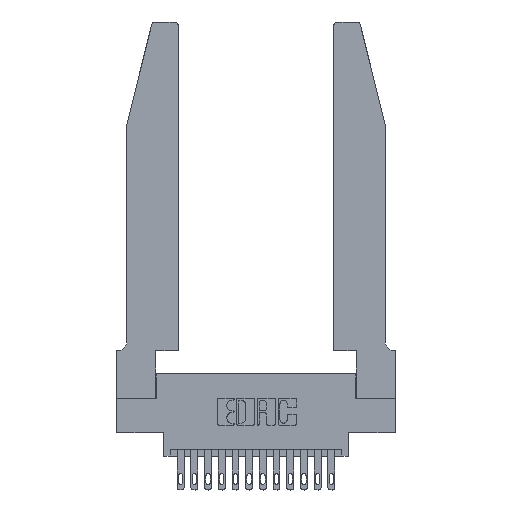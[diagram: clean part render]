
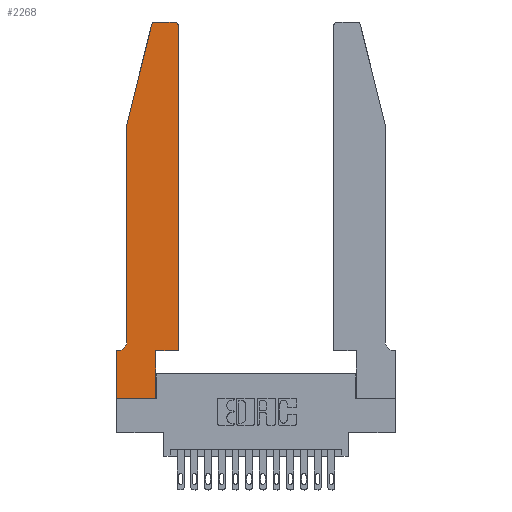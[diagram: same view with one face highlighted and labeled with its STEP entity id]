
A CAD part, top view. The second image highlights one B-rep face of the part: STEP entity #2268.
In plain terms, the highlighted planar face has unit normal (0, 0, 1).
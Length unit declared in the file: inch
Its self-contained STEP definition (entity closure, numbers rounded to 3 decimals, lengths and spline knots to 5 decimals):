
#92 = DIRECTION ( 'NONE',  ( 0., 0., 1. ) ) ;
#184 = ORIENTED_EDGE ( 'NONE', *, *, #8042, .T. ) ;
#872 = ORIENTED_EDGE ( 'NONE', *, *, #10988, .T. ) ;
#1040 = VECTOR ( 'NONE', #16801, 39.37008 ) ;
#1099 = DIRECTION ( 'NONE',  ( 1., 0., 0. ) ) ;
#1201 = EDGE_CURVE ( 'NONE', #16765, #8810, #13561, .T. ) ;
#1229 = DIRECTION ( 'NONE',  ( -1., 0., 0. ) ) ;
#1458 = DIRECTION ( 'NONE',  ( 1., 0., 0. ) ) ;
#1979 = AXIS2_PLACEMENT_3D ( 'NONE', #12449, #15235, #1229 ) ;
#2033 = EDGE_LOOP ( 'NONE', ( #11758, #17235, #184, #8457, #3432, #6998, #6655, #3687, #8711, #6825, #872, #7220 ) ) ;
#2268 = ADVANCED_FACE ( 'NONE', ( #6787 ), #9186, .T. ) ;
#2339 = EDGE_CURVE ( 'NONE', #12014, #3816, #12275, .T. ) ;
#2723 = CARTESIAN_POINT ( 'NONE',  ( 0.4205, 2.75, 0.37 ) ) ;
#2742 = CARTESIAN_POINT ( 'NONE',  ( 0.4505, 0.35, 0.37 ) ) ;
#2926 = EDGE_CURVE ( 'NONE', #8810, #10530, #14921, .T. ) ;
#3192 = AXIS2_PLACEMENT_3D ( 'NONE', #13345, #7558, #4908 ) ;
#3237 = AXIS2_PLACEMENT_3D ( 'NONE', #14167, #92, #1458 ) ;
#3383 = VECTOR ( 'NONE', #9747, 39.37008 ) ;
#3432 = ORIENTED_EDGE ( 'NONE', *, *, #2339, .T. ) ;
#3562 = CARTESIAN_POINT ( 'NONE',  ( 0.0755, 0.35, 0.37 ) ) ;
#3647 = CARTESIAN_POINT ( 'NONE',  ( 0., 0.35, 0.37 ) ) ;
#3648 = LINE ( 'NONE', #8197, #14235 ) ;
#3687 = ORIENTED_EDGE ( 'NONE', *, *, #1201, .T. ) ;
#3816 = VERTEX_POINT ( 'NONE', #4847 ) ;
#4797 = EDGE_CURVE ( 'NONE', #3816, #5520, #5380, .T. ) ;
#4847 = CARTESIAN_POINT ( 'NONE',  ( 0.0055, 0.35, 0.37 ) ) ;
#4908 = DIRECTION ( 'NONE',  ( 1., 0., 0. ) ) ;
#5380 = LINE ( 'NONE', #3562, #17283 ) ;
#5520 = VERTEX_POINT ( 'NONE', #7675 ) ;
#6226 = LINE ( 'NONE', #16584, #9998 ) ;
#6383 = DIRECTION ( 'NONE',  ( -1., 0., 0. ) ) ;
#6390 = EDGE_CURVE ( 'NONE', #12432, #17370, #14367, .T. ) ;
#6594 = DIRECTION ( 'NONE',  ( 0., 0., 1. ) ) ;
#6602 = VERTEX_POINT ( 'NONE', #9844 ) ;
#6655 = ORIENTED_EDGE ( 'NONE', *, *, #17991, .T. ) ;
#6787 = FACE_OUTER_BOUND ( 'NONE', #2033, .T. ) ;
#6825 = ORIENTED_EDGE ( 'NONE', *, *, #15756, .T. ) ;
#6895 = CARTESIAN_POINT ( 'NONE',  ( 0.2865, 0.35, 0.37 ) ) ;
#6998 = ORIENTED_EDGE ( 'NONE', *, *, #4797, .T. ) ;
#7220 = ORIENTED_EDGE ( 'NONE', *, *, #6390, .T. ) ;
#7558 = DIRECTION ( 'NONE',  ( 0., 0., 1. ) ) ;
#7675 = CARTESIAN_POINT ( 'NONE',  ( 0., 0.35, 0.37 ) ) ;
#8042 = EDGE_CURVE ( 'NONE', #8714, #6602, #9462, .T. ) ;
#8156 = DIRECTION ( 'NONE',  ( 1., 0., 0. ) ) ;
#8197 = CARTESIAN_POINT ( 'NONE',  ( 0.0755, 2., 0.37 ) ) ;
#8437 = DIRECTION ( 'NONE',  ( 0., -1., 0. ) ) ;
#8457 = ORIENTED_EDGE ( 'NONE', *, *, #12025, .T. ) ;
#8711 = ORIENTED_EDGE ( 'NONE', *, *, #2926, .T. ) ;
#8714 = VERTEX_POINT ( 'NONE', #14118 ) ;
#8810 = VERTEX_POINT ( 'NONE', #10510 ) ;
#9011 = CIRCLE ( 'NONE', #3237, 0.03 ) ;
#9186 = PLANE ( 'NONE',  #16751 ) ;
#9462 = LINE ( 'NONE', #15212, #17379 ) ;
#9611 = DIRECTION ( 'NONE',  ( 0., -1., 0. ) ) ;
#9747 = DIRECTION ( 'NONE',  ( 1., 0., 0. ) ) ;
#9813 = VECTOR ( 'NONE', #1099, 39.37008 ) ;
#9817 = EDGE_CURVE ( 'NONE', #14340, #8714, #9011, .T. ) ;
#9844 = CARTESIAN_POINT ( 'NONE',  ( 0.0755, 2., 0.37 ) ) ;
#9998 = VECTOR ( 'NONE', #12687, 39.37008 ) ;
#10510 = CARTESIAN_POINT ( 'NONE',  ( 0.2865, 0., 0.37 ) ) ;
#10530 = VERTEX_POINT ( 'NONE', #12834 ) ;
#10717 = DIRECTION ( 'NONE',  ( -0.239, -0.971, 0. ) ) ;
#10988 = EDGE_CURVE ( 'NONE', #16265, #12432, #12936, .T. ) ;
#11128 = CARTESIAN_POINT ( 'NONE',  ( 0., 0., 0.37 ) ) ;
#11173 = VECTOR ( 'NONE', #18281, 39.37008 ) ;
#11206 = CARTESIAN_POINT ( 'NONE',  ( 0., 0., 0.37 ) ) ;
#11302 = VECTOR ( 'NONE', #8437, 39.37008 ) ;
#11758 = ORIENTED_EDGE ( 'NONE', *, *, #14048, .T. ) ;
#12013 = CARTESIAN_POINT ( 'NONE',  ( 0.284, 2.75, 0.37 ) ) ;
#12014 = VERTEX_POINT ( 'NONE', #17066 ) ;
#12025 = EDGE_CURVE ( 'NONE', #6602, #12014, #3648, .T. ) ;
#12275 = CIRCLE ( 'NONE', #1979, 0.07 ) ;
#12432 = VERTEX_POINT ( 'NONE', #17805 ) ;
#12449 = CARTESIAN_POINT ( 'NONE',  ( 0.0055, 0.42, 0.37 ) ) ;
#12687 = DIRECTION ( 'NONE',  ( -1., 0., 0. ) ) ;
#12834 = CARTESIAN_POINT ( 'NONE',  ( 0.2865, 0.35, 0.37 ) ) ;
#12936 = LINE ( 'NONE', #2742, #1040 ) ;
#13345 = CARTESIAN_POINT ( 'NONE',  ( 0.4205, 2.72, 0.37 ) ) ;
#13561 = LINE ( 'NONE', #15042, #9813 ) ;
#13671 = CARTESIAN_POINT ( 'NONE',  ( 0.4505, 0.35, 0.37 ) ) ;
#14048 = EDGE_CURVE ( 'NONE', #17370, #14340, #6226, .T. ) ;
#14118 = CARTESIAN_POINT ( 'NONE',  ( 0.25487, 2.72718, 0.37 ) ) ;
#14167 = CARTESIAN_POINT ( 'NONE',  ( 0.284, 2.72, 0.37 ) ) ;
#14235 = VECTOR ( 'NONE', #9611, 39.37008 ) ;
#14340 = VERTEX_POINT ( 'NONE', #12013 ) ;
#14367 = CIRCLE ( 'NONE', #3192, 0.03 ) ;
#14396 = LINE ( 'NONE', #18189, #3383 ) ;
#14921 = LINE ( 'NONE', #6895, #11173 ) ;
#15042 = CARTESIAN_POINT ( 'NONE',  ( 0., 0., 0.37 ) ) ;
#15212 = CARTESIAN_POINT ( 'NONE',  ( 0.0755, 2., 0.37 ) ) ;
#15235 = DIRECTION ( 'NONE',  ( 0., 0., -1. ) ) ;
#15520 = LINE ( 'NONE', #11206, #11302 ) ;
#15756 = EDGE_CURVE ( 'NONE', #10530, #16265, #14396, .T. ) ;
#16265 = VERTEX_POINT ( 'NONE', #13671 ) ;
#16584 = CARTESIAN_POINT ( 'NONE',  ( 0.2605, 2.75, 0.37 ) ) ;
#16751 = AXIS2_PLACEMENT_3D ( 'NONE', #3647, #6594, #8156 ) ;
#16765 = VERTEX_POINT ( 'NONE', #11128 ) ;
#16801 = DIRECTION ( 'NONE',  ( 0., 1., 0. ) ) ;
#17066 = CARTESIAN_POINT ( 'NONE',  ( 0.0755, 0.42, 0.37 ) ) ;
#17235 = ORIENTED_EDGE ( 'NONE', *, *, #9817, .T. ) ;
#17283 = VECTOR ( 'NONE', #6383, 39.37008 ) ;
#17370 = VERTEX_POINT ( 'NONE', #2723 ) ;
#17379 = VECTOR ( 'NONE', #10717, 39.37008 ) ;
#17805 = CARTESIAN_POINT ( 'NONE',  ( 0.4505, 2.72, 0.37 ) ) ;
#17991 = EDGE_CURVE ( 'NONE', #5520, #16765, #15520, .T. ) ;
#18189 = CARTESIAN_POINT ( 'NONE',  ( 0.4505, 0.35, 0.37 ) ) ;
#18281 = DIRECTION ( 'NONE',  ( 0., 1., 0. ) ) ;
